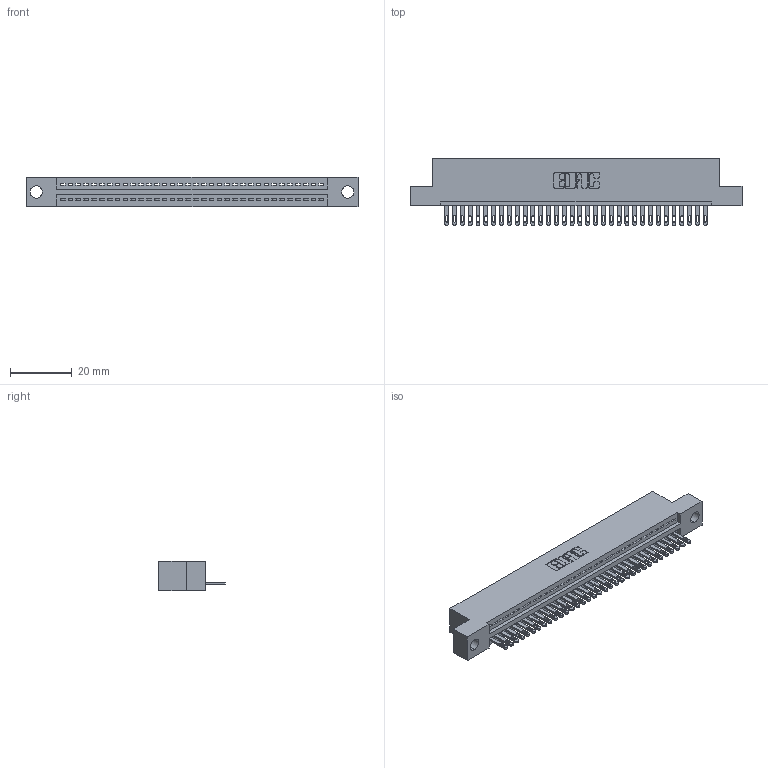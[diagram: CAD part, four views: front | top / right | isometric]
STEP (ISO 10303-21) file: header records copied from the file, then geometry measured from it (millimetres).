
FILE_DESCRIPTION (( 'STEP AP203' ), '1' );
FILE_NAME ('345-034-500-104.STEP', '2018-08-28T23:26:54', ( '' ), ( '' ), 'SwSTEP 2.0', 'SolidWorks 2016', '' );
FILE_SCHEMA (( 'CONFIG_CONTROL_DESIGN' ));
Length unit declared in the file: inch
Products named in the file (3): 345 Part_Flush Mounting Lugs - 0.156 Dia-TH; 345-292-001_345-293-100; 345-034-500-104
Assembly tree (35 placements, depth 2):
  345-034-500-104
    345 Part_Flush Mounting Lugs - 0.156 Dia-TH
    345-292-001_345-293-100  x34
Bounding box: 107.57 x 21.51 x 9.4 mm (x, y, z)
Volume: 10084.7 mm3; surface area: 13178 mm2
Topology: 35 solids, 35 shells, 1962 faces, 6053 edges, 4034 vertices
Faces by surface type: plane 1236, cylinder 726
Entity records: 26599 total; most frequent: CARTESIAN_POINT 4614, ORIENTED_EDGE 4582, DIRECTION 4043, EDGE_CURVE 2291, LINE 2019, VECTOR 2019, VERTEX_POINT 1526, AXIS2_PLACEMENT_3D 1012
